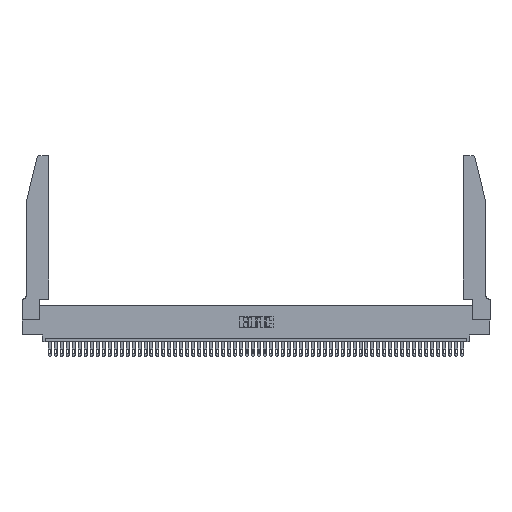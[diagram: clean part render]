
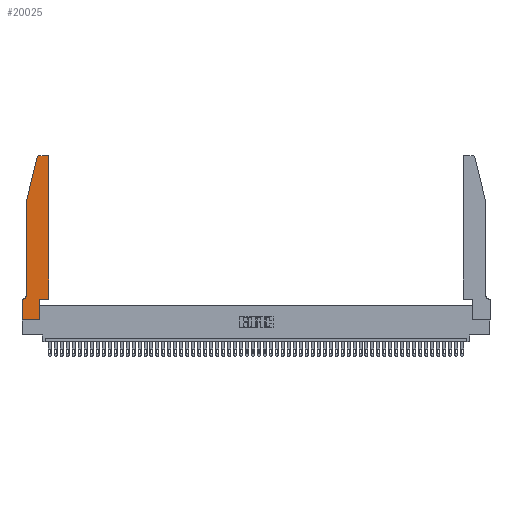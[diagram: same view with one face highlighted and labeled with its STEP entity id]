
A CAD part, top view. The second image highlights one B-rep face of the part: STEP entity #20025.
In plain terms, the highlighted planar face has unit normal (0, 0, 1).
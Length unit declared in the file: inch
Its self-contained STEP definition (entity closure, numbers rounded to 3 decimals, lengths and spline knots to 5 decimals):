
#92 = EDGE_CURVE ( 'NONE', #35790, #51696, #8523, .T. ) ;
#375 = EDGE_CURVE ( 'NONE', #11525, #12895, #13046, .T. ) ;
#942 = VERTEX_POINT ( 'NONE', #5274 ) ;
#1384 = AXIS2_PLACEMENT_3D ( 'NONE', #45566, #53409, #21211 ) ;
#1696 = PLANE ( 'NONE',  #8301 ) ;
#1800 = CARTESIAN_POINT ( 'NONE',  ( 0.284, 2.75, 0.37 ) ) ;
#1837 = CARTESIAN_POINT ( 'NONE',  ( 0.4505, 0.35, 0.37 ) ) ;
#2295 = LINE ( 'NONE', #43341, #3649 ) ;
#2361 = DIRECTION ( 'NONE',  ( 0., -1., 0. ) ) ;
#2629 = CARTESIAN_POINT ( 'NONE',  ( 0.284, 2.72, 0.37 ) ) ;
#3410 = DIRECTION ( 'NONE',  ( 0., -1., 0. ) ) ;
#3649 = VECTOR ( 'NONE', #2361, 39.37008 ) ;
#5214 = VECTOR ( 'NONE', #41892, 39.37008 ) ;
#5274 = CARTESIAN_POINT ( 'NONE',  ( 0., 0., 0.37 ) ) ;
#5304 = ORIENTED_EDGE ( 'NONE', *, *, #17079, .T. ) ;
#5597 = VERTEX_POINT ( 'NONE', #48724 ) ;
#5998 = CARTESIAN_POINT ( 'NONE',  ( 0.0755, 0.42, 0.37 ) ) ;
#6086 = LINE ( 'NONE', #14663, #9962 ) ;
#6439 = CARTESIAN_POINT ( 'NONE',  ( 0.4205, 2.75, 0.37 ) ) ;
#6963 = AXIS2_PLACEMENT_3D ( 'NONE', #2629, #15029, #39448 ) ;
#7024 = ORIENTED_EDGE ( 'NONE', *, *, #51423, .T. ) ;
#7233 = AXIS2_PLACEMENT_3D ( 'NONE', #15310, #52606, #48993 ) ;
#8243 = VERTEX_POINT ( 'NONE', #31526 ) ;
#8301 = AXIS2_PLACEMENT_3D ( 'NONE', #22798, #48034, #52958 ) ;
#8523 = LINE ( 'NONE', #50025, #5214 ) ;
#9330 = CARTESIAN_POINT ( 'NONE',  ( 0., 0.35, 0.37 ) ) ;
#9962 = VECTOR ( 'NONE', #10245, 39.37008 ) ;
#10245 = DIRECTION ( 'NONE',  ( -1., 0., 0. ) ) ;
#10489 = VECTOR ( 'NONE', #14408, 39.37008 ) ;
#11144 = VECTOR ( 'NONE', #3410, 39.37008 ) ;
#11417 = CARTESIAN_POINT ( 'NONE',  ( 0., 0., 0.37 ) ) ;
#11525 = VERTEX_POINT ( 'NONE', #43504 ) ;
#12122 = DIRECTION ( 'NONE',  ( 1., 0., 0. ) ) ;
#12293 = LINE ( 'NONE', #19959, #11144 ) ;
#12895 = VERTEX_POINT ( 'NONE', #1837 ) ;
#13046 = LINE ( 'NONE', #27893, #39642 ) ;
#13485 = VECTOR ( 'NONE', #51025, 39.37008 ) ;
#14408 = DIRECTION ( 'NONE',  ( 0., 1., 0. ) ) ;
#14663 = CARTESIAN_POINT ( 'NONE',  ( 0.2605, 2.75, 0.37 ) ) ;
#15029 = DIRECTION ( 'NONE',  ( 0., 0., 1. ) ) ;
#15310 = CARTESIAN_POINT ( 'NONE',  ( 0.4205, 2.72, 0.37 ) ) ;
#16029 = VERTEX_POINT ( 'NONE', #5998 ) ;
#16170 = VERTEX_POINT ( 'NONE', #38897 ) ;
#17079 = EDGE_CURVE ( 'NONE', #51696, #942, #12293, .T. ) ;
#18490 = EDGE_CURVE ( 'NONE', #50105, #16029, #2295, .T. ) ;
#18729 = LINE ( 'NONE', #34181, #13485 ) ;
#19789 = LINE ( 'NONE', #11417, #44449 ) ;
#19959 = CARTESIAN_POINT ( 'NONE',  ( 0., 0., 0.37 ) ) ;
#20025 = ADVANCED_FACE ( 'NONE', ( #41130 ), #1696, .T. ) ;
#20448 = ORIENTED_EDGE ( 'NONE', *, *, #21912, .T. ) ;
#21211 = DIRECTION ( 'NONE',  ( -1., 0., 0. ) ) ;
#21912 = EDGE_CURVE ( 'NONE', #8243, #11525, #51268, .T. ) ;
#21914 = VERTEX_POINT ( 'NONE', #1800 ) ;
#22629 = VECTOR ( 'NONE', #32753, 39.37008 ) ;
#22726 = CARTESIAN_POINT ( 'NONE',  ( 0.0055, 0.35, 0.37 ) ) ;
#22798 = CARTESIAN_POINT ( 'NONE',  ( 0., 0.35, 0.37 ) ) ;
#23996 = LINE ( 'NONE', #31793, #22629 ) ;
#24445 = EDGE_CURVE ( 'NONE', #12895, #5597, #18729, .T. ) ;
#24742 = ORIENTED_EDGE ( 'NONE', *, *, #375, .T. ) ;
#24929 = ORIENTED_EDGE ( 'NONE', *, *, #18490, .T. ) ;
#26731 = ORIENTED_EDGE ( 'NONE', *, *, #32362, .T. ) ;
#27893 = CARTESIAN_POINT ( 'NONE',  ( 0.4505, 0.35, 0.37 ) ) ;
#28937 = CIRCLE ( 'NONE', #7233, 0.03 ) ;
#29647 = CARTESIAN_POINT ( 'NONE',  ( 0.0755, 2., 0.37 ) ) ;
#29903 = ORIENTED_EDGE ( 'NONE', *, *, #30270, .T. ) ;
#30262 = CIRCLE ( 'NONE', #1384, 0.07 ) ;
#30270 = EDGE_CURVE ( 'NONE', #942, #8243, #19789, .T. ) ;
#31526 = CARTESIAN_POINT ( 'NONE',  ( 0.2865, 0., 0.37 ) ) ;
#31793 = CARTESIAN_POINT ( 'NONE',  ( 0.0755, 2., 0.37 ) ) ;
#32207 = ORIENTED_EDGE ( 'NONE', *, *, #92, .T. ) ;
#32362 = EDGE_CURVE ( 'NONE', #21914, #16170, #49381, .T. ) ;
#32753 = DIRECTION ( 'NONE',  ( -0.239, -0.971, 0. ) ) ;
#34181 = CARTESIAN_POINT ( 'NONE',  ( 0.4505, 0.35, 0.37 ) ) ;
#34514 = EDGE_LOOP ( 'NONE', ( #41595, #26731, #53260, #24929, #35255, #32207, #5304, #29903, #20448, #24742, #45717, #7024 ) ) ;
#35255 = ORIENTED_EDGE ( 'NONE', *, *, #38543, .T. ) ;
#35790 = VERTEX_POINT ( 'NONE', #22726 ) ;
#36748 = EDGE_CURVE ( 'NONE', #16170, #50105, #23996, .T. ) ;
#38543 = EDGE_CURVE ( 'NONE', #16029, #35790, #30262, .T. ) ;
#38897 = CARTESIAN_POINT ( 'NONE',  ( 0.25487, 2.72718, 0.37 ) ) ;
#39448 = DIRECTION ( 'NONE',  ( 1., 0., 0. ) ) ;
#39642 = VECTOR ( 'NONE', #52546, 39.37008 ) ;
#41130 = FACE_OUTER_BOUND ( 'NONE', #34514, .T. ) ;
#41595 = ORIENTED_EDGE ( 'NONE', *, *, #47011, .T. ) ;
#41892 = DIRECTION ( 'NONE',  ( -1., 0., 0. ) ) ;
#43010 = CARTESIAN_POINT ( 'NONE',  ( 0.2865, 0.35, 0.37 ) ) ;
#43341 = CARTESIAN_POINT ( 'NONE',  ( 0.0755, 2., 0.37 ) ) ;
#43504 = CARTESIAN_POINT ( 'NONE',  ( 0.2865, 0.35, 0.37 ) ) ;
#44449 = VECTOR ( 'NONE', #12122, 39.37008 ) ;
#44512 = VERTEX_POINT ( 'NONE', #6439 ) ;
#45566 = CARTESIAN_POINT ( 'NONE',  ( 0.0055, 0.42, 0.37 ) ) ;
#45717 = ORIENTED_EDGE ( 'NONE', *, *, #24445, .T. ) ;
#47011 = EDGE_CURVE ( 'NONE', #44512, #21914, #6086, .T. ) ;
#48034 = DIRECTION ( 'NONE',  ( 0., 0., 1. ) ) ;
#48724 = CARTESIAN_POINT ( 'NONE',  ( 0.4505, 2.72, 0.37 ) ) ;
#48993 = DIRECTION ( 'NONE',  ( 1., 0., 0. ) ) ;
#49381 = CIRCLE ( 'NONE', #6963, 0.03 ) ;
#50025 = CARTESIAN_POINT ( 'NONE',  ( 0.0755, 0.35, 0.37 ) ) ;
#50105 = VERTEX_POINT ( 'NONE', #29647 ) ;
#51025 = DIRECTION ( 'NONE',  ( 0., 1., 0. ) ) ;
#51268 = LINE ( 'NONE', #43010, #10489 ) ;
#51423 = EDGE_CURVE ( 'NONE', #5597, #44512, #28937, .T. ) ;
#51696 = VERTEX_POINT ( 'NONE', #9330 ) ;
#52546 = DIRECTION ( 'NONE',  ( 1., 0., 0. ) ) ;
#52606 = DIRECTION ( 'NONE',  ( 0., 0., 1. ) ) ;
#52958 = DIRECTION ( 'NONE',  ( 1., 0., 0. ) ) ;
#53260 = ORIENTED_EDGE ( 'NONE', *, *, #36748, .T. ) ;
#53409 = DIRECTION ( 'NONE',  ( 0., 0., -1. ) ) ;
